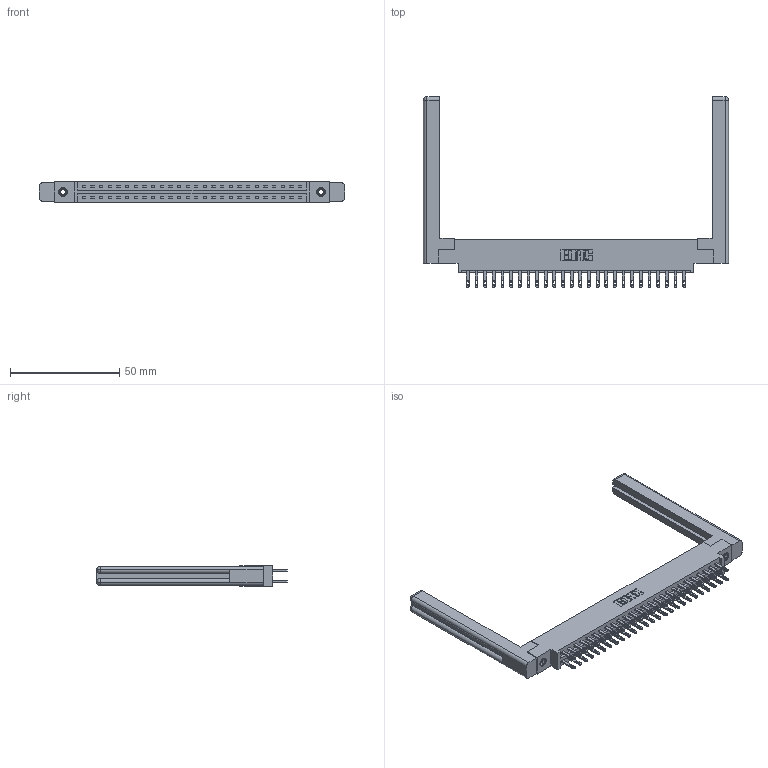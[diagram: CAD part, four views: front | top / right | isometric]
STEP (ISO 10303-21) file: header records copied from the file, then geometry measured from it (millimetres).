
FILE_DESCRIPTION (( 'STEP AP203' ), '1' );
FILE_NAME ('337-052-500-858.STEP', '2019-10-11T17:59:34', ( '' ), ( '' ), 'SwSTEP 2.0', 'SolidWorks 2016', '' );
FILE_SCHEMA (( 'CONFIG_CONTROL_DESIGN' ));
Length unit declared in the file: inch
Products named in the file (5): 337-052-500-858; 345-250-001_345-250-001-102; 307-220-058; 337 Part_0.170 Offset - 0.156 Dia-TI; 345-292-001_345-293-100
Assembly tree (57 placements, depth 2):
  337-052-500-858
    337 Part_0.170 Offset - 0.156 Dia-TI
    345-292-001_345-293-100  x52
    345-250-001_345-250-001-102  x2
    307-220-058  x2
Bounding box: 139.65 x 87.25 x 9.4 mm (x, y, z)
Volume: 21688.1 mm3; surface area: 22020.2 mm2
Topology: 57 solids, 57 shells, 2860 faces, 8633 edges, 5742 vertices
Faces by surface type: plane 1822, cylinder 1014, cone 12, torus 12
Entity records: 24924 total; most frequent: CARTESIAN_POINT 4221, ORIENTED_EDGE 4096, DIRECTION 3636, EDGE_CURVE 2048, VECTOR 1868, LINE 1868, VERTEX_POINT 1358, AXIS2_PLACEMENT_3D 884
